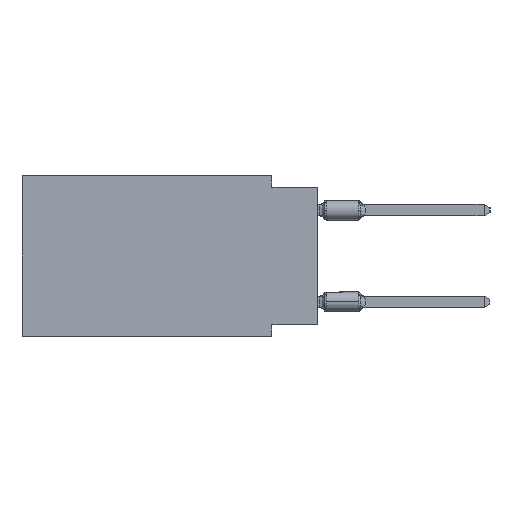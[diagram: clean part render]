
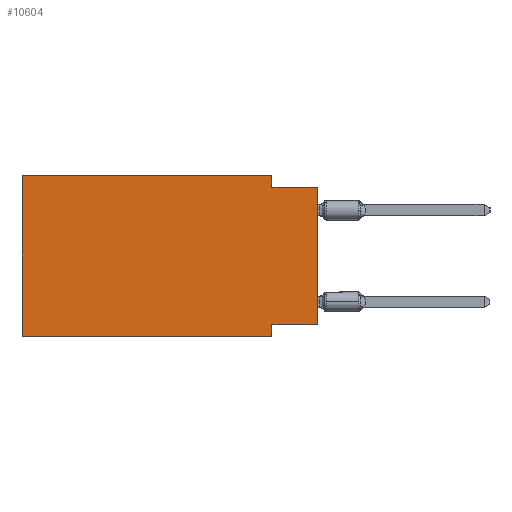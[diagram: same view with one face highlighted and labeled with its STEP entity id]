
A CAD part, left-side view. The second image highlights one B-rep face of the part: STEP entity #10604.
In plain terms, the highlighted planar face has unit normal (-1, 0, 0).
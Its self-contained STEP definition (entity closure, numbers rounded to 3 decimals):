
#1267 = VERTEX_POINT ( 'NONE', #31551 ) ;
#1553 = EDGE_CURVE ( 'NONE', #41106, #36550, #9594, .T. ) ;
#2436 = CARTESIAN_POINT ( 'NONE',  ( 0., 16.383, 0. ) ) ;
#4255 = ORIENTED_EDGE ( 'NONE', *, *, #36720, .F. ) ;
#5644 = CARTESIAN_POINT ( 'NONE',  ( 0., 2.54, 0. ) ) ;
#6020 = EDGE_CURVE ( 'NONE', #10966, #31504, #9319, .T. ) ;
#6247 = ORIENTED_EDGE ( 'NONE', *, *, #24617, .T. ) ;
#6749 = DIRECTION ( 'NONE',  ( 0., 1., 0. ) ) ;
#6912 = LINE ( 'NONE', #24945, #29069 ) ;
#7337 = VERTEX_POINT ( 'NONE', #28745 ) ;
#7492 = ORIENTED_EDGE ( 'NONE', *, *, #44723, .T. ) ;
#7570 = EDGE_CURVE ( 'NONE', #12364, #7337, #33762, .T. ) ;
#9319 = LINE ( 'NONE', #5644, #12594 ) ;
#9594 = LINE ( 'NONE', #27196, #44781 ) ;
#9813 = VECTOR ( 'NONE', #43591, 1000. ) ;
#10604 = ADVANCED_FACE ( 'NONE', ( #39210 ), #11751, .F. ) ;
#10966 = VERTEX_POINT ( 'NONE', #25584 ) ;
#11751 = PLANE ( 'NONE',  #28008 ) ;
#12364 = VERTEX_POINT ( 'NONE', #15638 ) ;
#12594 = VECTOR ( 'NONE', #23486, 1000. ) ;
#12966 = DIRECTION ( 'NONE',  ( 0., 0., 1. ) ) ;
#13130 = EDGE_CURVE ( 'NONE', #31504, #34186, #23465, .T. ) ;
#13552 = ORIENTED_EDGE ( 'NONE', *, *, #1553, .F. ) ;
#15098 = VECTOR ( 'NONE', #6749, 1000. ) ;
#15638 = CARTESIAN_POINT ( 'NONE',  ( 0., 16.383, -8.89 ) ) ;
#15642 = ORIENTED_EDGE ( 'NONE', *, *, #44062, .F. ) ;
#15761 = CARTESIAN_POINT ( 'NONE',  ( 0., 16.383, -8.89 ) ) ;
#16667 = LINE ( 'NONE', #15761, #24310 ) ;
#18388 = DIRECTION ( 'NONE',  ( 1., 0., 0. ) ) ;
#18762 = LINE ( 'NONE', #38892, #35419 ) ;
#19890 = CARTESIAN_POINT ( 'NONE',  ( 0., 2.54, -0.635 ) ) ;
#21374 = CARTESIAN_POINT ( 'NONE',  ( 0., 0., -8.255 ) ) ;
#23465 = LINE ( 'NONE', #23695, #9813 ) ;
#23486 = DIRECTION ( 'NONE',  ( 0., 0., -1. ) ) ;
#23543 = DIRECTION ( 'NONE',  ( 0., 0., -1. ) ) ;
#23695 = CARTESIAN_POINT ( 'NONE',  ( 0., 0., -0.635 ) ) ;
#24310 = VECTOR ( 'NONE', #44335, 1000. ) ;
#24617 = EDGE_CURVE ( 'NONE', #1267, #34186, #18762, .T. ) ;
#24844 = ORIENTED_EDGE ( 'NONE', *, *, #6020, .F. ) ;
#24945 = CARTESIAN_POINT ( 'NONE',  ( 0., 16.383, 0. ) ) ;
#25584 = CARTESIAN_POINT ( 'NONE',  ( 0., 2.54, 0. ) ) ;
#27196 = CARTESIAN_POINT ( 'NONE',  ( 0., 2.54, -8.89 ) ) ;
#28008 = AXIS2_PLACEMENT_3D ( 'NONE', #28234, #18388, #38988 ) ;
#28234 = CARTESIAN_POINT ( 'NONE',  ( 0., 16.383, 0. ) ) ;
#28524 = VECTOR ( 'NONE', #12966, 1000. ) ;
#28745 = CARTESIAN_POINT ( 'NONE',  ( 0., 16.383, 0. ) ) ;
#29040 = DIRECTION ( 'NONE',  ( 0., 0., 1. ) ) ;
#29069 = VECTOR ( 'NONE', #31804, 1000. ) ;
#31504 = VERTEX_POINT ( 'NONE', #19890 ) ;
#31551 = CARTESIAN_POINT ( 'NONE',  ( 0., 0., -8.255 ) ) ;
#31804 = DIRECTION ( 'NONE',  ( 0., -1., 0. ) ) ;
#31849 = EDGE_LOOP ( 'NONE', ( #6247, #37189, #24844, #15642, #41157, #7492, #13552, #4255 ) ) ;
#33762 = LINE ( 'NONE', #2436, #28524 ) ;
#34186 = VERTEX_POINT ( 'NONE', #41231 ) ;
#35419 = VECTOR ( 'NONE', #29040, 1000. ) ;
#36550 = VERTEX_POINT ( 'NONE', #36767 ) ;
#36720 = EDGE_CURVE ( 'NONE', #1267, #41106, #42188, .T. ) ;
#36767 = CARTESIAN_POINT ( 'NONE',  ( 0., 2.54, -8.89 ) ) ;
#37189 = ORIENTED_EDGE ( 'NONE', *, *, #13130, .F. ) ;
#38892 = CARTESIAN_POINT ( 'NONE',  ( 0., 0., 0. ) ) ;
#38988 = DIRECTION ( 'NONE',  ( 0., 0., -1. ) ) ;
#39210 = FACE_OUTER_BOUND ( 'NONE', #31849, .T. ) ;
#40025 = CARTESIAN_POINT ( 'NONE',  ( 0., 2.54, -8.255 ) ) ;
#41106 = VERTEX_POINT ( 'NONE', #40025 ) ;
#41157 = ORIENTED_EDGE ( 'NONE', *, *, #7570, .F. ) ;
#41231 = CARTESIAN_POINT ( 'NONE',  ( 0., 0., -0.635 ) ) ;
#42188 = LINE ( 'NONE', #21374, #15098 ) ;
#43591 = DIRECTION ( 'NONE',  ( 0., -1., 0. ) ) ;
#44062 = EDGE_CURVE ( 'NONE', #7337, #10966, #6912, .T. ) ;
#44335 = DIRECTION ( 'NONE',  ( 0., -1., 0. ) ) ;
#44723 = EDGE_CURVE ( 'NONE', #12364, #36550, #16667, .T. ) ;
#44781 = VECTOR ( 'NONE', #23543, 1000. ) ;
